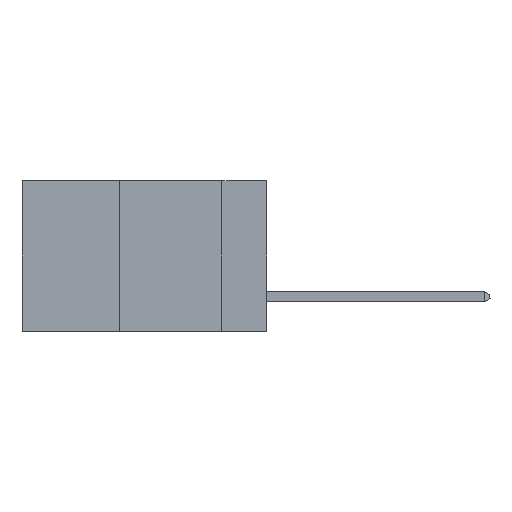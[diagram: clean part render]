
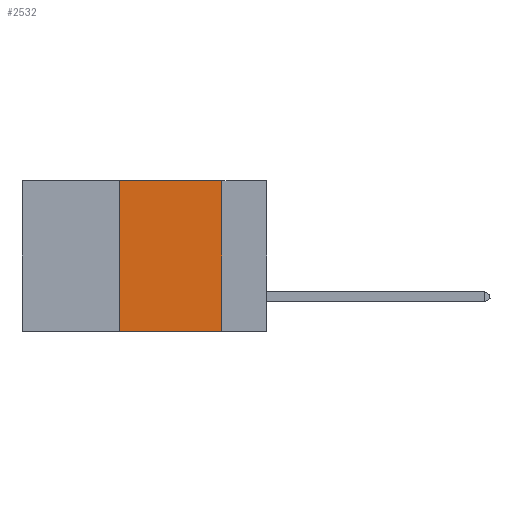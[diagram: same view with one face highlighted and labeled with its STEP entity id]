
A CAD part, left-side view. The second image highlights one B-rep face of the part: STEP entity #2532.
In plain terms, the highlighted planar face has unit normal (-1, 0, 0).
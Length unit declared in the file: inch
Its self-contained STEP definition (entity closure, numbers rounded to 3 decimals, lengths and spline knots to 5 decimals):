
#159 = LINE ( 'NONE', #7333, #15305 ) ;
#160 = DIRECTION ( 'NONE',  ( 0., -1., 0. ) ) ;
#1882 = CARTESIAN_POINT ( 'NONE',  ( 0., 0.6, 0. ) ) ;
#1889 = VECTOR ( 'NONE', #23551, 39.37008 ) ;
#1971 = EDGE_CURVE ( 'NONE', #2519, #6567, #28115, .T. ) ;
#2519 = VERTEX_POINT ( 'NONE', #15665 ) ;
#2532 = ADVANCED_FACE ( 'NONE', ( #24439 ), #11230, .F. ) ;
#3515 = VERTEX_POINT ( 'NONE', #22302 ) ;
#3838 = CARTESIAN_POINT ( 'NONE',  ( 0., 0.6, 0. ) ) ;
#4328 = AXIS2_PLACEMENT_3D ( 'NONE', #1882, #17982, #20318 ) ;
#5354 = ORIENTED_EDGE ( 'NONE', *, *, #23216, .F. ) ;
#5980 = VECTOR ( 'NONE', #160, 39.37008 ) ;
#6567 = VERTEX_POINT ( 'NONE', #27239 ) ;
#7333 = CARTESIAN_POINT ( 'NONE',  ( 0., 0.11, 0. ) ) ;
#7390 = CARTESIAN_POINT ( 'NONE',  ( 0., 0.36, 0. ) ) ;
#8589 = ORIENTED_EDGE ( 'NONE', *, *, #21913, .F. ) ;
#9294 = CARTESIAN_POINT ( 'NONE',  ( 0., 0.6, -0.37 ) ) ;
#10749 = DIRECTION ( 'NONE',  ( 0., -1., 0. ) ) ;
#11230 = PLANE ( 'NONE',  #4328 ) ;
#14068 = LINE ( 'NONE', #7390, #1889 ) ;
#15044 = ORIENTED_EDGE ( 'NONE', *, *, #21246, .T. ) ;
#15305 = VECTOR ( 'NONE', #28261, 39.37008 ) ;
#15665 = CARTESIAN_POINT ( 'NONE',  ( 0., 0.36, 0. ) ) ;
#17502 = LINE ( 'NONE', #9294, #5980 ) ;
#17982 = DIRECTION ( 'NONE',  ( 1., 0., 0. ) ) ;
#18138 = EDGE_LOOP ( 'NONE', ( #8589, #22385, #5354, #15044 ) ) ;
#20318 = DIRECTION ( 'NONE',  ( 0., 0., -1. ) ) ;
#20395 = VERTEX_POINT ( 'NONE', #22108 ) ;
#21246 = EDGE_CURVE ( 'NONE', #3515, #20395, #17502, .T. ) ;
#21913 = EDGE_CURVE ( 'NONE', #6567, #20395, #159, .T. ) ;
#22108 = CARTESIAN_POINT ( 'NONE',  ( 0., 0.11, -0.37 ) ) ;
#22302 = CARTESIAN_POINT ( 'NONE',  ( 0., 0.36, -0.37 ) ) ;
#22385 = ORIENTED_EDGE ( 'NONE', *, *, #1971, .F. ) ;
#23216 = EDGE_CURVE ( 'NONE', #3515, #2519, #14068, .T. ) ;
#23551 = DIRECTION ( 'NONE',  ( 0., 0., 1. ) ) ;
#24439 = FACE_OUTER_BOUND ( 'NONE', #18138, .T. ) ;
#27025 = VECTOR ( 'NONE', #10749, 39.37008 ) ;
#27239 = CARTESIAN_POINT ( 'NONE',  ( 0., 0.11, 0. ) ) ;
#28115 = LINE ( 'NONE', #3838, #27025 ) ;
#28261 = DIRECTION ( 'NONE',  ( 0., 0., -1. ) ) ;
